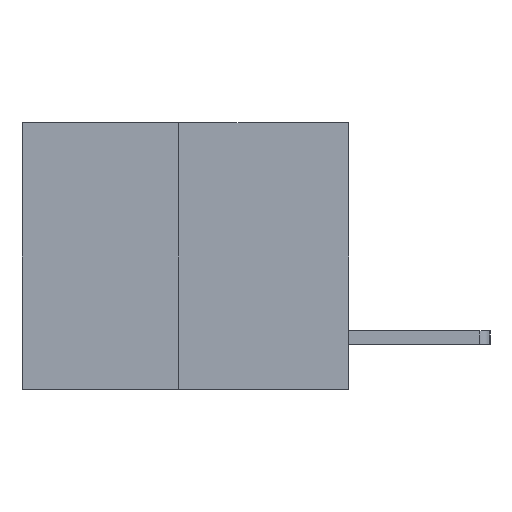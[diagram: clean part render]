
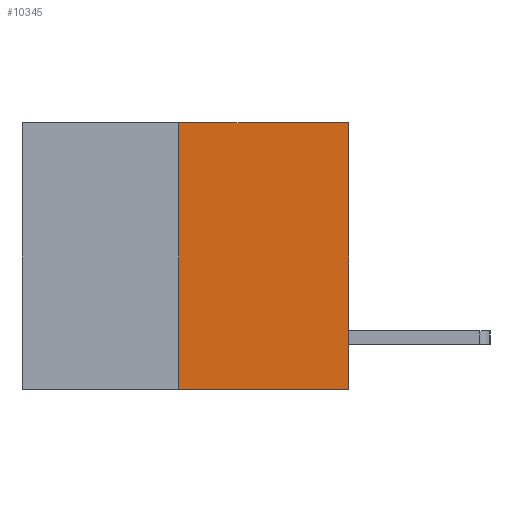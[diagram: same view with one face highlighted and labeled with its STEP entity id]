
A CAD part, left-side view. The second image highlights one B-rep face of the part: STEP entity #10345.
In plain terms, the highlighted planar face has unit normal (-1, 0, 0).
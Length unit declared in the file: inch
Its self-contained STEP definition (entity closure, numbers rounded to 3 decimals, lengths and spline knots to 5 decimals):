
#786 = FACE_OUTER_BOUND ( 'NONE', #9743, .T. ) ;
#829 = ORIENTED_EDGE ( 'NONE', *, *, #5135, .T. ) ;
#1121 = ORIENTED_EDGE ( 'NONE', *, *, #2651, .F. ) ;
#1405 = CARTESIAN_POINT ( 'NONE',  ( 0., 0.312, -0.49 ) ) ;
#1425 = VERTEX_POINT ( 'NONE', #9259 ) ;
#1471 = CARTESIAN_POINT ( 'NONE',  ( 0., 0., 0. ) ) ;
#1500 = VECTOR ( 'NONE', #4793, 39.37008 ) ;
#1867 = DIRECTION ( 'NONE',  ( 0., 0., 1. ) ) ;
#2012 = ORIENTED_EDGE ( 'NONE', *, *, #10591, .T. ) ;
#2232 = VERTEX_POINT ( 'NONE', #10191 ) ;
#2651 = EDGE_CURVE ( 'NONE', #1425, #10013, #3492, .T. ) ;
#2741 = DIRECTION ( 'NONE',  ( 0., -1., 0. ) ) ;
#3360 = VECTOR ( 'NONE', #11137, 39.37008 ) ;
#3492 = LINE ( 'NONE', #8867, #5684 ) ;
#3566 = VECTOR ( 'NONE', #1867, 39.37008 ) ;
#4422 = CARTESIAN_POINT ( 'NONE',  ( 0., 0., 0. ) ) ;
#4583 = LINE ( 'NONE', #9490, #3360 ) ;
#4584 = DIRECTION ( 'NONE',  ( 0., 0., -1. ) ) ;
#4778 = AXIS2_PLACEMENT_3D ( 'NONE', #6365, #8181, #4584 ) ;
#4793 = DIRECTION ( 'NONE',  ( 0., 0., 1. ) ) ;
#5135 = EDGE_CURVE ( 'NONE', #2232, #10013, #9503, .T. ) ;
#5586 = PLANE ( 'NONE',  #4778 ) ;
#5684 = VECTOR ( 'NONE', #2741, 39.37008 ) ;
#6365 = CARTESIAN_POINT ( 'NONE',  ( 0., 0.6, 0. ) ) ;
#6527 = EDGE_CURVE ( 'NONE', #8425, #1425, #7518, .T. ) ;
#7518 = LINE ( 'NONE', #10126, #1500 ) ;
#7997 = ORIENTED_EDGE ( 'NONE', *, *, #6527, .F. ) ;
#8181 = DIRECTION ( 'NONE',  ( 1., 0., 0. ) ) ;
#8425 = VERTEX_POINT ( 'NONE', #1405 ) ;
#8867 = CARTESIAN_POINT ( 'NONE',  ( 0., 0.6, 0. ) ) ;
#9259 = CARTESIAN_POINT ( 'NONE',  ( 0., 0.312, 0. ) ) ;
#9490 = CARTESIAN_POINT ( 'NONE',  ( 0., 0.6, -0.49 ) ) ;
#9503 = LINE ( 'NONE', #4422, #3566 ) ;
#9743 = EDGE_LOOP ( 'NONE', ( #7997, #2012, #829, #1121 ) ) ;
#10013 = VERTEX_POINT ( 'NONE', #1471 ) ;
#10126 = CARTESIAN_POINT ( 'NONE',  ( 0., 0.312, -0.49 ) ) ;
#10191 = CARTESIAN_POINT ( 'NONE',  ( 0., 0., -0.49 ) ) ;
#10345 = ADVANCED_FACE ( 'NONE', ( #786 ), #5586, .F. ) ;
#10591 = EDGE_CURVE ( 'NONE', #8425, #2232, #4583, .T. ) ;
#11137 = DIRECTION ( 'NONE',  ( 0., -1., 0. ) ) ;
